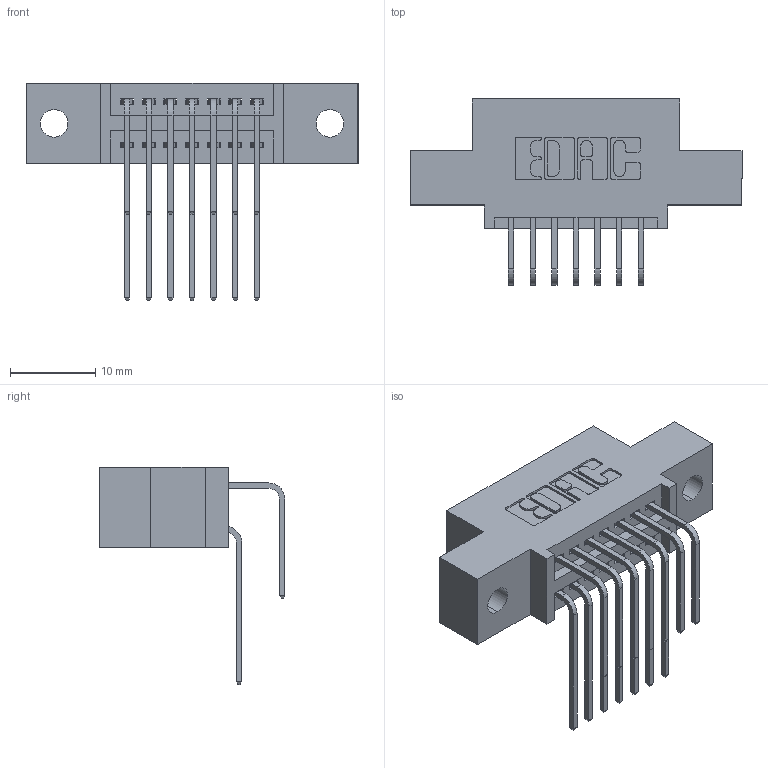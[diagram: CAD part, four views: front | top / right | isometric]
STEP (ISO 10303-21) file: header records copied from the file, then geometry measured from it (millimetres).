
FILE_DESCRIPTION (( 'STEP AP203' ), '1' );
FILE_NAME ('395-014-558-502.STEP', '2019-10-15T16:52:29', ( '' ), ( '' ), 'SwSTEP 2.0', 'SolidWorks 2016', '' );
FILE_SCHEMA (( 'CONFIG_CONTROL_DESIGN' ));
Length unit declared in the file: inch
Products named in the file (4): 345 Part_0.110 Offset - 0.128 Dia; 345-292-001_558 559 Tail - 1; 345-292-001_558 Tail - 2; 395-014-558-502
Assembly tree (15 placements, depth 2):
  395-014-558-502
    345 Part_0.110 Offset - 0.128 Dia
    345-292-001_558 559 Tail - 1  x7
    345-292-001_558 Tail - 2  x7
Bounding box: 38.99 x 21.83 x 25.53 mm (x, y, z)
Volume: 3433.3 mm3; surface area: 4596.9 mm2
Topology: 15 solids, 15 shells, 858 faces, 2523 edges, 1662 vertices
Faces by surface type: plane 574, cylinder 284
Entity records: 11991 total; most frequent: CARTESIAN_POINT 2091, ORIENTED_EDGE 1974, DIRECTION 1859, EDGE_CURVE 987, VECTOR 787, LINE 787, VERTEX_POINT 654, AXIS2_PLACEMENT_3D 536
